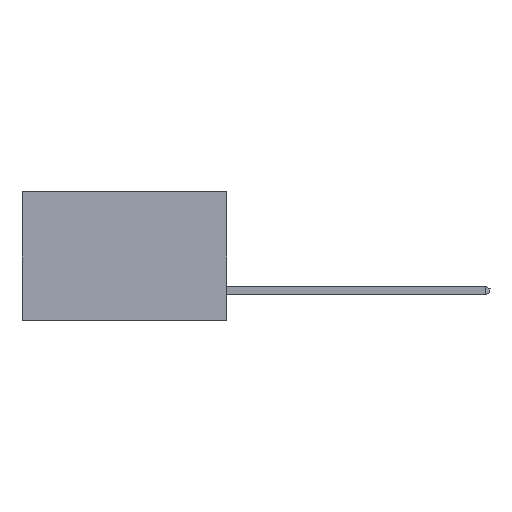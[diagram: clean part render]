
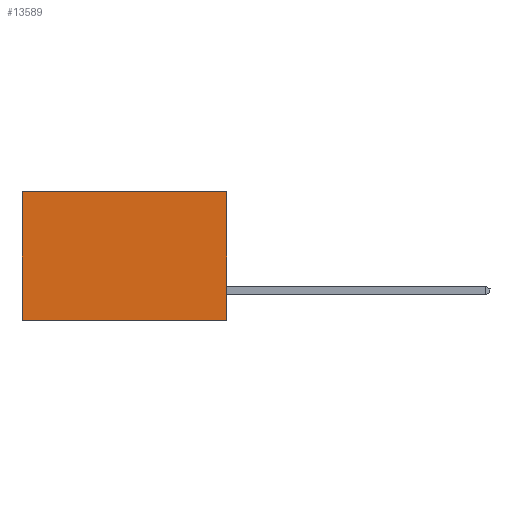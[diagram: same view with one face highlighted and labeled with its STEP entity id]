
A CAD part, left-side view. The second image highlights one B-rep face of the part: STEP entity #13589.
In plain terms, the highlighted planar face has unit normal (-1, 0, 0).
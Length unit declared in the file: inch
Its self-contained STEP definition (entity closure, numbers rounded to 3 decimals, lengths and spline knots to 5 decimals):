
#141 = CARTESIAN_POINT ( 'NONE',  ( 0.277, 0.59, 0. ) ) ;
#446 = DIRECTION ( 'NONE',  ( 0., 1., 0. ) ) ;
#527 = ORIENTED_EDGE ( 'NONE', *, *, #8296, .T. ) ;
#547 = CARTESIAN_POINT ( 'NONE',  ( 0.277, 0., 0. ) ) ;
#1062 = LINE ( 'NONE', #1424, #9839 ) ;
#1173 = VECTOR ( 'NONE', #446, 39.37008 ) ;
#1393 = DIRECTION ( 'NONE',  ( 0., 1., 0. ) ) ;
#1424 = CARTESIAN_POINT ( 'NONE',  ( 0.277, 0., -0.37 ) ) ;
#1626 = VERTEX_POINT ( 'NONE', #6972 ) ;
#1956 = LINE ( 'NONE', #9129, #13251 ) ;
#2274 = EDGE_LOOP ( 'NONE', ( #10082, #2470, #4343, #527 ) ) ;
#2470 = ORIENTED_EDGE ( 'NONE', *, *, #5204, .F. ) ;
#3638 = VERTEX_POINT ( 'NONE', #141 ) ;
#3987 = VERTEX_POINT ( 'NONE', #4626 ) ;
#4024 = PLANE ( 'NONE',  #8782 ) ;
#4343 = ORIENTED_EDGE ( 'NONE', *, *, #12247, .F. ) ;
#4626 = CARTESIAN_POINT ( 'NONE',  ( 0.277, 0.59, -0.37 ) ) ;
#5204 = EDGE_CURVE ( 'NONE', #1626, #3987, #1062, .T. ) ;
#5387 = DIRECTION ( 'NONE',  ( 0., 0., -1. ) ) ;
#6081 = FACE_OUTER_BOUND ( 'NONE', #2274, .T. ) ;
#6972 = CARTESIAN_POINT ( 'NONE',  ( 0.277, 0., -0.37 ) ) ;
#7429 = DIRECTION ( 'NONE',  ( 0., 0., -1. ) ) ;
#7637 = CARTESIAN_POINT ( 'NONE',  ( 0.277, 0., -0.37 ) ) ;
#8296 = EDGE_CURVE ( 'NONE', #11598, #3638, #12923, .T. ) ;
#8782 = AXIS2_PLACEMENT_3D ( 'NONE', #12677, #13675, #7429 ) ;
#9129 = CARTESIAN_POINT ( 'NONE',  ( 0.277, 0.59, -0.37 ) ) ;
#9839 = VECTOR ( 'NONE', #1393, 39.37008 ) ;
#10082 = ORIENTED_EDGE ( 'NONE', *, *, #12454, .T. ) ;
#10221 = DIRECTION ( 'NONE',  ( 0., 0., -1. ) ) ;
#11108 = VECTOR ( 'NONE', #5387, 39.37008 ) ;
#11598 = VERTEX_POINT ( 'NONE', #13779 ) ;
#12247 = EDGE_CURVE ( 'NONE', #11598, #1626, #13726, .T. ) ;
#12454 = EDGE_CURVE ( 'NONE', #3638, #3987, #1956, .T. ) ;
#12677 = CARTESIAN_POINT ( 'NONE',  ( 0.277, 0., -0.37 ) ) ;
#12923 = LINE ( 'NONE', #547, #1173 ) ;
#13251 = VECTOR ( 'NONE', #10221, 39.37008 ) ;
#13589 = ADVANCED_FACE ( 'NONE', ( #6081 ), #4024, .F. ) ;
#13675 = DIRECTION ( 'NONE',  ( 1., 0., 0. ) ) ;
#13726 = LINE ( 'NONE', #7637, #11108 ) ;
#13779 = CARTESIAN_POINT ( 'NONE',  ( 0.277, 0., 0. ) ) ;
